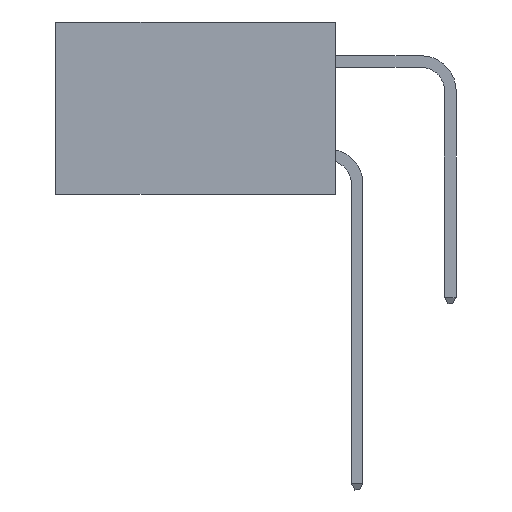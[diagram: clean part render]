
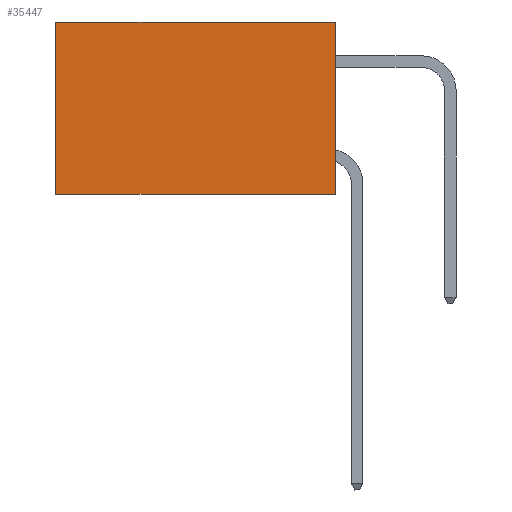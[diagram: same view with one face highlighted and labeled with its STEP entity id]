
A CAD part, left-side view. The second image highlights one B-rep face of the part: STEP entity #35447.
In plain terms, the highlighted planar face has unit normal (-1, 0, 0).
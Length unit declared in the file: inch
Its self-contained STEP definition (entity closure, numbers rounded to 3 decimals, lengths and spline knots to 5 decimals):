
#3526 = ORIENTED_EDGE ( 'NONE', *, *, #5283, .T. ) ;
#5283 = EDGE_CURVE ( 'NONE', #22236, #18540, #28927, .T. ) ;
#5777 = CARTESIAN_POINT ( 'NONE',  ( 0.2875, 0., 0. ) ) ;
#5799 = FACE_OUTER_BOUND ( 'NONE', #37474, .T. ) ;
#6100 = DIRECTION ( 'NONE',  ( 0., 1., 0. ) ) ;
#6788 = CARTESIAN_POINT ( 'NONE',  ( 0.2875, 0., 0. ) ) ;
#7813 = VECTOR ( 'NONE', #27837, 39.37008 ) ;
#7930 = LINE ( 'NONE', #5777, #19397 ) ;
#11536 = LINE ( 'NONE', #27630, #13458 ) ;
#12289 = EDGE_CURVE ( 'NONE', #17534, #18540, #11536, .T. ) ;
#13458 = VECTOR ( 'NONE', #6100, 39.37008 ) ;
#14266 = CARTESIAN_POINT ( 'NONE',  ( 0.2875, 0., -0.37 ) ) ;
#14879 = PLANE ( 'NONE',  #34295 ) ;
#16885 = CARTESIAN_POINT ( 'NONE',  ( 0.2875, 0.6, 0. ) ) ;
#17175 = CARTESIAN_POINT ( 'NONE',  ( 0.2875, 0.6, 0. ) ) ;
#17211 = VERTEX_POINT ( 'NONE', #6788 ) ;
#17534 = VERTEX_POINT ( 'NONE', #14266 ) ;
#17947 = DIRECTION ( 'NONE',  ( 1., 0., 0. ) ) ;
#18035 = ORIENTED_EDGE ( 'NONE', *, *, #12289, .F. ) ;
#18540 = VERTEX_POINT ( 'NONE', #37250 ) ;
#19397 = VECTOR ( 'NONE', #24897, 39.37008 ) ;
#21130 = ORIENTED_EDGE ( 'NONE', *, *, #29932, .F. ) ;
#21966 = ORIENTED_EDGE ( 'NONE', *, *, #33290, .T. ) ;
#22236 = VERTEX_POINT ( 'NONE', #16885 ) ;
#24072 = DIRECTION ( 'NONE',  ( 0., 0., -1. ) ) ;
#24897 = DIRECTION ( 'NONE',  ( 0., 1., 0. ) ) ;
#27285 = CARTESIAN_POINT ( 'NONE',  ( 0.2875, 0., 0. ) ) ;
#27630 = CARTESIAN_POINT ( 'NONE',  ( 0.2875, 0., -0.37 ) ) ;
#27837 = DIRECTION ( 'NONE',  ( 0., 0., -1. ) ) ;
#27907 = LINE ( 'NONE', #30631, #7813 ) ;
#28927 = LINE ( 'NONE', #17175, #30827 ) ;
#29844 = DIRECTION ( 'NONE',  ( 0., 0., -1. ) ) ;
#29932 = EDGE_CURVE ( 'NONE', #17211, #17534, #27907, .T. ) ;
#30631 = CARTESIAN_POINT ( 'NONE',  ( 0.2875, 0., 0. ) ) ;
#30827 = VECTOR ( 'NONE', #29844, 39.37008 ) ;
#33290 = EDGE_CURVE ( 'NONE', #17211, #22236, #7930, .T. ) ;
#34295 = AXIS2_PLACEMENT_3D ( 'NONE', #27285, #17947, #24072 ) ;
#35447 = ADVANCED_FACE ( 'NONE', ( #5799 ), #14879, .F. ) ;
#37250 = CARTESIAN_POINT ( 'NONE',  ( 0.2875, 0.6, -0.37 ) ) ;
#37474 = EDGE_LOOP ( 'NONE', ( #3526, #18035, #21130, #21966 ) ) ;
